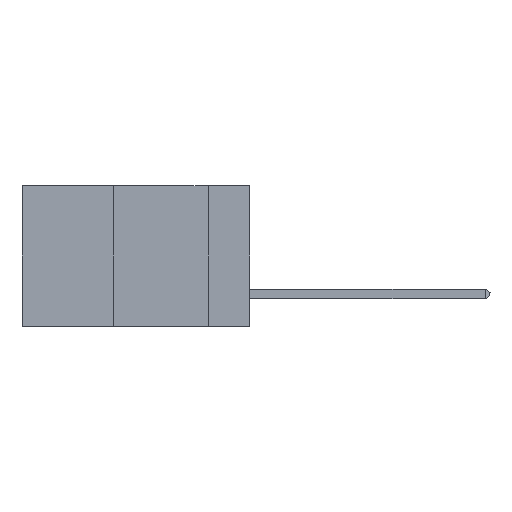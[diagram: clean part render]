
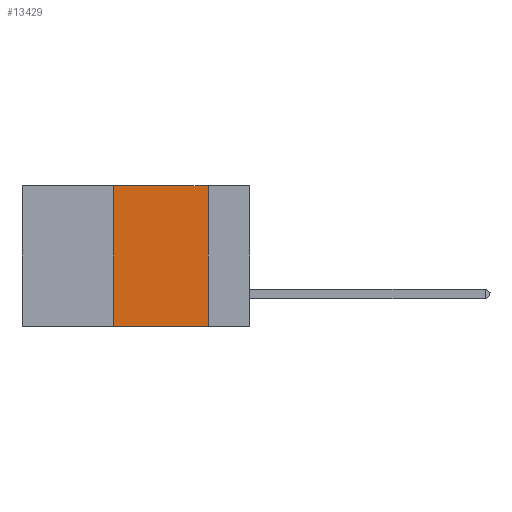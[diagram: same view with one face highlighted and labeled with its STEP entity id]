
A CAD part, left-side view. The second image highlights one B-rep face of the part: STEP entity #13429.
In plain terms, the highlighted planar face has unit normal (-1, 0, 0).
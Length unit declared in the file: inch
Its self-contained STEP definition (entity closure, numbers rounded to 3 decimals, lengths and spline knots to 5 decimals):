
#1168 = CARTESIAN_POINT ( 'NONE',  ( 0., 0.11, 0. ) ) ;
#1618 = EDGE_CURVE ( 'NONE', #22752, #25121, #30306, .T. ) ;
#2377 = DIRECTION ( 'NONE',  ( 1., 0., 0. ) ) ;
#2806 = LINE ( 'NONE', #1168, #34694 ) ;
#3822 = EDGE_CURVE ( 'NONE', #25121, #20912, #9881, .T. ) ;
#7542 = CARTESIAN_POINT ( 'NONE',  ( 0., 0.11, -0.37 ) ) ;
#9169 = AXIS2_PLACEMENT_3D ( 'NONE', #23096, #2377, #30374 ) ;
#9881 = LINE ( 'NONE', #14730, #15769 ) ;
#13429 = ADVANCED_FACE ( 'NONE', ( #38040 ), #30221, .F. ) ;
#14730 = CARTESIAN_POINT ( 'NONE',  ( 0., 0.6, 0. ) ) ;
#14967 = CARTESIAN_POINT ( 'NONE',  ( 0., 0.36, -0.37 ) ) ;
#15769 = VECTOR ( 'NONE', #36974, 39.37008 ) ;
#16261 = CARTESIAN_POINT ( 'NONE',  ( 0., 0.36, 0. ) ) ;
#20046 = VECTOR ( 'NONE', #37397, 39.37008 ) ;
#20912 = VERTEX_POINT ( 'NONE', #22886 ) ;
#20969 = ORIENTED_EDGE ( 'NONE', *, *, #42311, .F. ) ;
#21696 = EDGE_LOOP ( 'NONE', ( #20969, #21971, #36296, #29227 ) ) ;
#21971 = ORIENTED_EDGE ( 'NONE', *, *, #3822, .F. ) ;
#22752 = VERTEX_POINT ( 'NONE', #14967 ) ;
#22886 = CARTESIAN_POINT ( 'NONE',  ( 0., 0.11, 0. ) ) ;
#23096 = CARTESIAN_POINT ( 'NONE',  ( 0., 0.6, 0. ) ) ;
#25121 = VERTEX_POINT ( 'NONE', #16261 ) ;
#25352 = VERTEX_POINT ( 'NONE', #7542 ) ;
#28277 = LINE ( 'NONE', #32045, #35859 ) ;
#28424 = DIRECTION ( 'NONE',  ( 0., -1., 0. ) ) ;
#29227 = ORIENTED_EDGE ( 'NONE', *, *, #40376, .T. ) ;
#30221 = PLANE ( 'NONE',  #9169 ) ;
#30306 = LINE ( 'NONE', #32987, #20046 ) ;
#30374 = DIRECTION ( 'NONE',  ( 0., 0., -1. ) ) ;
#32045 = CARTESIAN_POINT ( 'NONE',  ( 0., 0.6, -0.37 ) ) ;
#32987 = CARTESIAN_POINT ( 'NONE',  ( 0., 0.36, 0. ) ) ;
#34694 = VECTOR ( 'NONE', #39467, 39.37008 ) ;
#35859 = VECTOR ( 'NONE', #28424, 39.37008 ) ;
#36296 = ORIENTED_EDGE ( 'NONE', *, *, #1618, .F. ) ;
#36974 = DIRECTION ( 'NONE',  ( 0., -1., 0. ) ) ;
#37397 = DIRECTION ( 'NONE',  ( 0., 0., 1. ) ) ;
#38040 = FACE_OUTER_BOUND ( 'NONE', #21696, .T. ) ;
#39467 = DIRECTION ( 'NONE',  ( 0., 0., -1. ) ) ;
#40376 = EDGE_CURVE ( 'NONE', #22752, #25352, #28277, .T. ) ;
#42311 = EDGE_CURVE ( 'NONE', #20912, #25352, #2806, .T. ) ;
